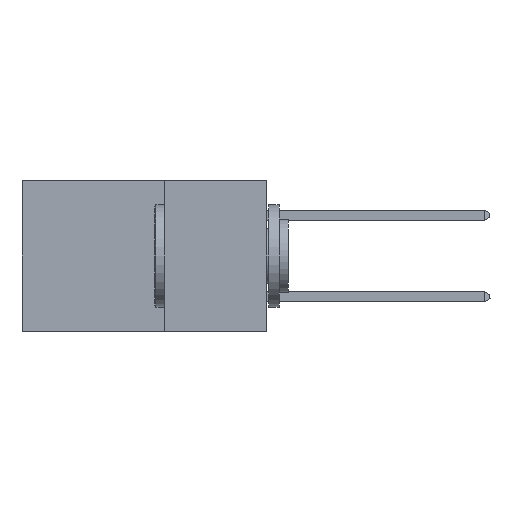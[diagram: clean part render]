
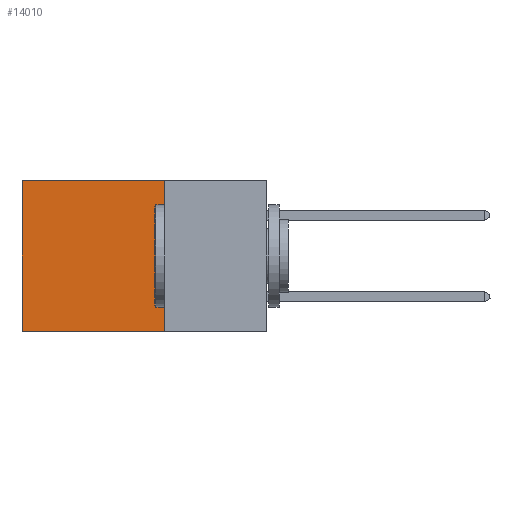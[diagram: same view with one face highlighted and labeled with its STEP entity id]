
A CAD part, left-side view. The second image highlights one B-rep face of the part: STEP entity #14010.
In plain terms, the highlighted planar face has unit normal (-1, 0, 0).
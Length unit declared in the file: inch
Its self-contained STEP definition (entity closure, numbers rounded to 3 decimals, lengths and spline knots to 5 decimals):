
#235 = EDGE_CURVE ( 'NONE', #19522, #4960, #21664, .T. ) ;
#264 = CARTESIAN_POINT ( 'NONE',  ( 0.2875, 0.25, 0. ) ) ;
#267 = LINE ( 'NONE', #26322, #6220 ) ;
#3776 = VECTOR ( 'NONE', #32140, 39.37008 ) ;
#4841 = ORIENTED_EDGE ( 'NONE', *, *, #24975, .T. ) ;
#4960 = VERTEX_POINT ( 'NONE', #32829 ) ;
#6220 = VECTOR ( 'NONE', #18730, 39.37008 ) ;
#6850 = ORIENTED_EDGE ( 'NONE', *, *, #20261, .T. ) ;
#7466 = VECTOR ( 'NONE', #10322, 39.37008 ) ;
#8182 = LINE ( 'NONE', #13184, #27343 ) ;
#9146 = CARTESIAN_POINT ( 'NONE',  ( 0.2875, 0.6, 0. ) ) ;
#9160 = VERTEX_POINT ( 'NONE', #9146 ) ;
#10322 = DIRECTION ( 'NONE',  ( 0., 1., 0. ) ) ;
#12771 = AXIS2_PLACEMENT_3D ( 'NONE', #21513, #14123, #31709 ) ;
#13184 = CARTESIAN_POINT ( 'NONE',  ( 0.2875, 0.25, -0.37 ) ) ;
#13799 = PLANE ( 'NONE',  #12771 ) ;
#14010 = ADVANCED_FACE ( 'NONE', ( #27494 ), #13799, .F. ) ;
#14123 = DIRECTION ( 'NONE',  ( 1., 0., 0. ) ) ;
#15952 = CARTESIAN_POINT ( 'NONE',  ( 0.2875, 0.6, -0.37 ) ) ;
#16342 = EDGE_LOOP ( 'NONE', ( #6850, #30975, #22551, #4841 ) ) ;
#18105 = CARTESIAN_POINT ( 'NONE',  ( 0.2875, 0.25, 0. ) ) ;
#18730 = DIRECTION ( 'NONE',  ( 0., 0., -1. ) ) ;
#19522 = VERTEX_POINT ( 'NONE', #18105 ) ;
#20207 = LINE ( 'NONE', #264, #7466 ) ;
#20261 = EDGE_CURVE ( 'NONE', #9160, #31316, #267, .T. ) ;
#20645 = EDGE_CURVE ( 'NONE', #4960, #31316, #8182, .T. ) ;
#21513 = CARTESIAN_POINT ( 'NONE',  ( 0.2875, 0.25, 0. ) ) ;
#21664 = LINE ( 'NONE', #29687, #3776 ) ;
#22551 = ORIENTED_EDGE ( 'NONE', *, *, #235, .F. ) ;
#24975 = EDGE_CURVE ( 'NONE', #19522, #9160, #20207, .T. ) ;
#26322 = CARTESIAN_POINT ( 'NONE',  ( 0.2875, 0.6, 0. ) ) ;
#27343 = VECTOR ( 'NONE', #28673, 39.37008 ) ;
#27494 = FACE_OUTER_BOUND ( 'NONE', #16342, .T. ) ;
#28673 = DIRECTION ( 'NONE',  ( 0., 1., 0. ) ) ;
#29687 = CARTESIAN_POINT ( 'NONE',  ( 0.2875, 0.25, 0. ) ) ;
#30975 = ORIENTED_EDGE ( 'NONE', *, *, #20645, .F. ) ;
#31316 = VERTEX_POINT ( 'NONE', #15952 ) ;
#31709 = DIRECTION ( 'NONE',  ( 0., 0., -1. ) ) ;
#32140 = DIRECTION ( 'NONE',  ( 0., 0., -1. ) ) ;
#32829 = CARTESIAN_POINT ( 'NONE',  ( 0.2875, 0.25, -0.37 ) ) ;
